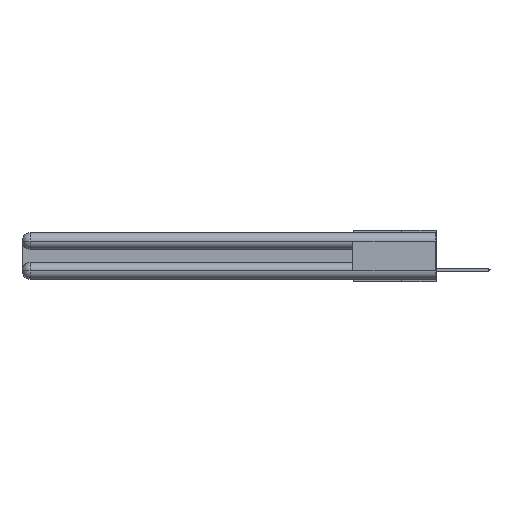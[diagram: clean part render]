
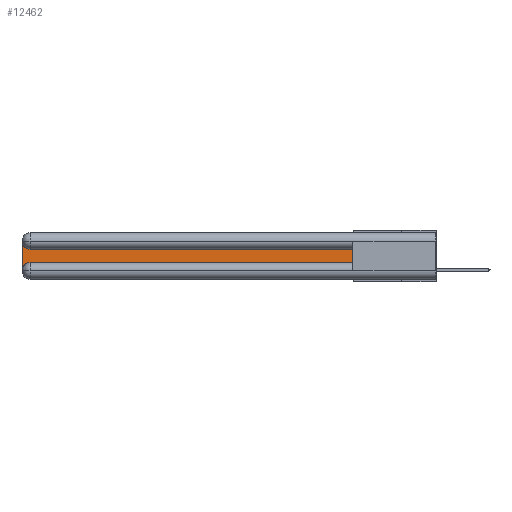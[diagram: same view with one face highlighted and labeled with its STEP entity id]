
A CAD part, left-side view. The second image highlights one B-rep face of the part: STEP entity #12462.
In plain terms, the highlighted planar face has unit normal (-1, 0, 0).
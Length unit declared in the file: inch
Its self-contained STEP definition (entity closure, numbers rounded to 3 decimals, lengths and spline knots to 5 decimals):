
#252 = EDGE_LOOP ( 'NONE', ( #14417, #14356, #30000, #22576, #24485, #25850 ) ) ;
#753 = EDGE_CURVE ( 'NONE', #12414, #21157, #3615, .T. ) ;
#1339 = CARTESIAN_POINT ( 'NONE',  ( 0.075, 2.94, -0.2175 ) ) ;
#1611 = CARTESIAN_POINT ( 'NONE',  ( 0.075, 3., -0.0625 ) ) ;
#1627 = AXIS2_PLACEMENT_3D ( 'NONE', #11892, #24570, #24791 ) ;
#3074 = DIRECTION ( 'NONE',  ( 0., 0., -1. ) ) ;
#3615 = CIRCLE ( 'NONE', #27380, 0.06 ) ;
#4253 = DIRECTION ( 'NONE',  ( 1., 0., 0. ) ) ;
#5190 = EDGE_CURVE ( 'NONE', #12447, #9269, #27117, .T. ) ;
#7061 = CARTESIAN_POINT ( 'NONE',  ( 0.075, 3., -0.1225 ) ) ;
#7634 = EDGE_CURVE ( 'NONE', #24430, #12447, #32943, .T. ) ;
#9269 = VERTEX_POINT ( 'NONE', #30695 ) ;
#10363 = AXIS2_PLACEMENT_3D ( 'NONE', #7061, #4253, #16972 ) ;
#10483 = DIRECTION ( 'NONE',  ( 0., 0., 1. ) ) ;
#10600 = DIRECTION ( 'NONE',  ( 1., 0., 0. ) ) ;
#11892 = CARTESIAN_POINT ( 'NONE',  ( 0.075, 2.94, -0.0625 ) ) ;
#12414 = VERTEX_POINT ( 'NONE', #24229 ) ;
#12447 = VERTEX_POINT ( 'NONE', #14854 ) ;
#12462 = ADVANCED_FACE ( 'NONE', ( #15020 ), #19622, .F. ) ;
#13433 = LINE ( 'NONE', #29418, #15850 ) ;
#13515 = EDGE_CURVE ( 'NONE', #15421, #12414, #19700, .T. ) ;
#14105 = CARTESIAN_POINT ( 'NONE',  ( 0.075, 3., -0.2175 ) ) ;
#14356 = ORIENTED_EDGE ( 'NONE', *, *, #14400, .T. ) ;
#14400 = EDGE_CURVE ( 'NONE', #9269, #15421, #22459, .T. ) ;
#14417 = ORIENTED_EDGE ( 'NONE', *, *, #5190, .T. ) ;
#14544 = CARTESIAN_POINT ( 'NONE',  ( 0.075, 0.6, -0.1225 ) ) ;
#14854 = CARTESIAN_POINT ( 'NONE',  ( 0.075, 0.6, -0.1225 ) ) ;
#15020 = FACE_OUTER_BOUND ( 'NONE', #252, .T. ) ;
#15421 = VERTEX_POINT ( 'NONE', #1611 ) ;
#15850 = VECTOR ( 'NONE', #29966, 39.37008 ) ;
#16972 = DIRECTION ( 'NONE',  ( 0., 0., -1. ) ) ;
#17502 = VECTOR ( 'NONE', #32448, 39.37008 ) ;
#18455 = CARTESIAN_POINT ( 'NONE',  ( 0.075, 2.94, -0.2775 ) ) ;
#19622 = PLANE ( 'NONE',  #10363 ) ;
#19700 = LINE ( 'NONE', #14105, #31750 ) ;
#21157 = VERTEX_POINT ( 'NONE', #1339 ) ;
#22459 = CIRCLE ( 'NONE', #1627, 0.06 ) ;
#22576 = ORIENTED_EDGE ( 'NONE', *, *, #753, .T. ) ;
#24229 = CARTESIAN_POINT ( 'NONE',  ( 0.075, 3., -0.2775 ) ) ;
#24348 = EDGE_CURVE ( 'NONE', #21157, #24430, #13433, .T. ) ;
#24430 = VERTEX_POINT ( 'NONE', #32207 ) ;
#24485 = ORIENTED_EDGE ( 'NONE', *, *, #24348, .T. ) ;
#24570 = DIRECTION ( 'NONE',  ( 1., 0., 0. ) ) ;
#24791 = DIRECTION ( 'NONE',  ( 0., 0., -1. ) ) ;
#25850 = ORIENTED_EDGE ( 'NONE', *, *, #7634, .T. ) ;
#26518 = VECTOR ( 'NONE', #10483, 39.37008 ) ;
#27117 = LINE ( 'NONE', #14544, #17502 ) ;
#27380 = AXIS2_PLACEMENT_3D ( 'NONE', #18455, #10600, #3074 ) ;
#28327 = CARTESIAN_POINT ( 'NONE',  ( 0.075, 0.6, -0.2175 ) ) ;
#29418 = CARTESIAN_POINT ( 'NONE',  ( 0.075, 0.6, -0.2175 ) ) ;
#29966 = DIRECTION ( 'NONE',  ( 0., -1., 0. ) ) ;
#30000 = ORIENTED_EDGE ( 'NONE', *, *, #13515, .T. ) ;
#30695 = CARTESIAN_POINT ( 'NONE',  ( 0.075, 2.94, -0.1225 ) ) ;
#31750 = VECTOR ( 'NONE', #31887, 39.37008 ) ;
#31887 = DIRECTION ( 'NONE',  ( 0., 0., -1. ) ) ;
#32207 = CARTESIAN_POINT ( 'NONE',  ( 0.075, 0.6, -0.2175 ) ) ;
#32448 = DIRECTION ( 'NONE',  ( 0., 1., 0. ) ) ;
#32943 = LINE ( 'NONE', #28327, #26518 ) ;
